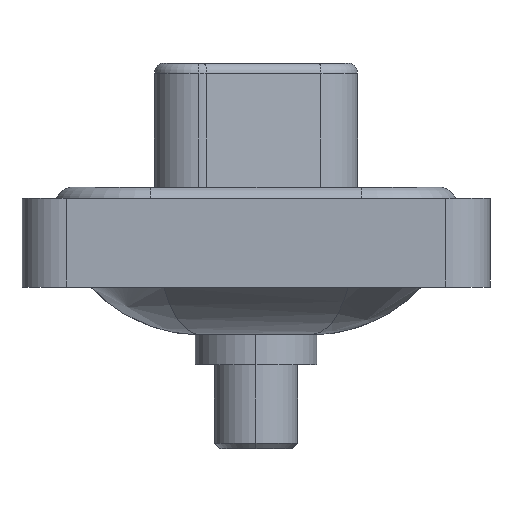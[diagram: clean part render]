
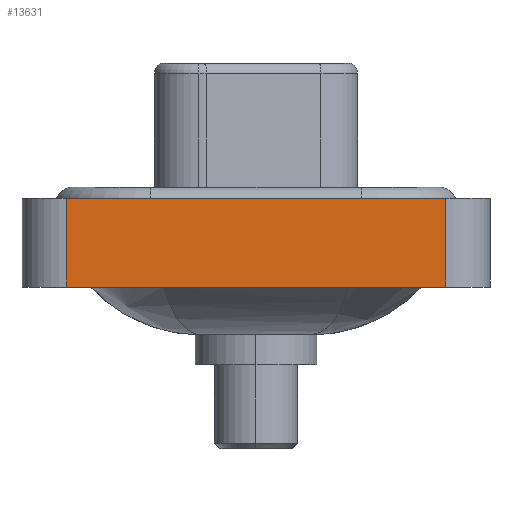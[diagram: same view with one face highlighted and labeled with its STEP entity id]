
A CAD part, left-side view. The second image highlights one B-rep face of the part: STEP entity #13631.
In plain terms, the highlighted planar face has unit normal (-1, 0, 0).
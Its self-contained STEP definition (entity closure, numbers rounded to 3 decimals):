
#252 = LINE ( 'NONE', #15643, #1171 ) ;
#1171 = VECTOR ( 'NONE', #11692, 1000. ) ;
#1565 = LINE ( 'NONE', #2925, #6923 ) ;
#2452 = ORIENTED_EDGE ( 'NONE', *, *, #10161, .F. ) ;
#2925 = CARTESIAN_POINT ( 'NONE',  ( -7.3, -8.55, -3.6 ) ) ;
#3821 = AXIS2_PLACEMENT_3D ( 'NONE', #11084, #13450, #11177 ) ;
#3823 = LINE ( 'NONE', #14232, #9711 ) ;
#4153 = PLANE ( 'NONE',  #3821 ) ;
#4189 = ORIENTED_EDGE ( 'NONE', *, *, #7938, .T. ) ;
#4965 = EDGE_LOOP ( 'NONE', ( #9378, #12331, #2452, #4189 ) ) ;
#5723 = VERTEX_POINT ( 'NONE', #13199 ) ;
#6522 = DIRECTION ( 'NONE',  ( 0., 0., 1. ) ) ;
#6923 = VECTOR ( 'NONE', #11813, 1000. ) ;
#6978 = VERTEX_POINT ( 'NONE', #12875 ) ;
#7938 = EDGE_CURVE ( 'NONE', #5723, #6978, #1565, .T. ) ;
#8425 = CARTESIAN_POINT ( 'NONE',  ( -7.3, 8.55, 0.4 ) ) ;
#9176 = VERTEX_POINT ( 'NONE', #8425 ) ;
#9378 = ORIENTED_EDGE ( 'NONE', *, *, #14598, .T. ) ;
#9581 = LINE ( 'NONE', #9738, #12646 ) ;
#9711 = VECTOR ( 'NONE', #6522, 1000. ) ;
#9738 = CARTESIAN_POINT ( 'NONE',  ( -7.3, 8.55, -3.6 ) ) ;
#10161 = EDGE_CURVE ( 'NONE', #5723, #9176, #9581, .T. ) ;
#11084 = CARTESIAN_POINT ( 'NONE',  ( -7.3, -8.55, -3.6 ) ) ;
#11177 = DIRECTION ( 'NONE',  ( 0., 0., 1. ) ) ;
#11692 = DIRECTION ( 'NONE',  ( 0., -1., 0. ) ) ;
#11813 = DIRECTION ( 'NONE',  ( 0., -1., 0. ) ) ;
#12299 = EDGE_CURVE ( 'NONE', #9176, #14213, #252, .T. ) ;
#12331 = ORIENTED_EDGE ( 'NONE', *, *, #12299, .F. ) ;
#12646 = VECTOR ( 'NONE', #14557, 1000. ) ;
#12875 = CARTESIAN_POINT ( 'NONE',  ( -7.3, -8.55, -3.6 ) ) ;
#13199 = CARTESIAN_POINT ( 'NONE',  ( -7.3, 8.55, -3.6 ) ) ;
#13450 = DIRECTION ( 'NONE',  ( -1., 0., 0. ) ) ;
#13631 = ADVANCED_FACE ( 'NONE', ( #15730 ), #4153, .T. ) ;
#14213 = VERTEX_POINT ( 'NONE', #15277 ) ;
#14232 = CARTESIAN_POINT ( 'NONE',  ( -7.3, -8.55, -3.6 ) ) ;
#14557 = DIRECTION ( 'NONE',  ( 0., 0., 1. ) ) ;
#14598 = EDGE_CURVE ( 'NONE', #6978, #14213, #3823, .T. ) ;
#15277 = CARTESIAN_POINT ( 'NONE',  ( -7.3, -8.55, 0.4 ) ) ;
#15643 = CARTESIAN_POINT ( 'NONE',  ( -7.3, -8.55, 0.4 ) ) ;
#15730 = FACE_OUTER_BOUND ( 'NONE', #4965, .T. ) ;
